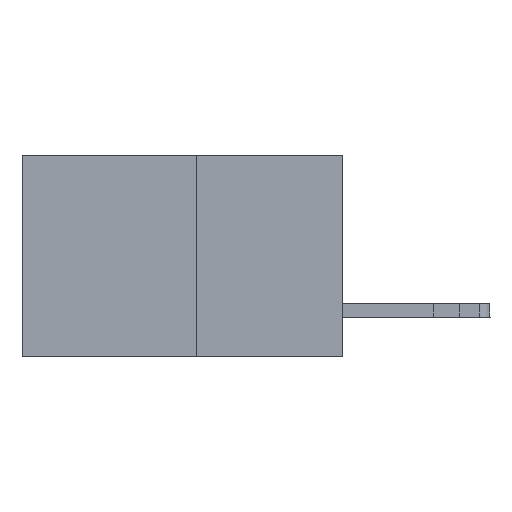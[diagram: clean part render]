
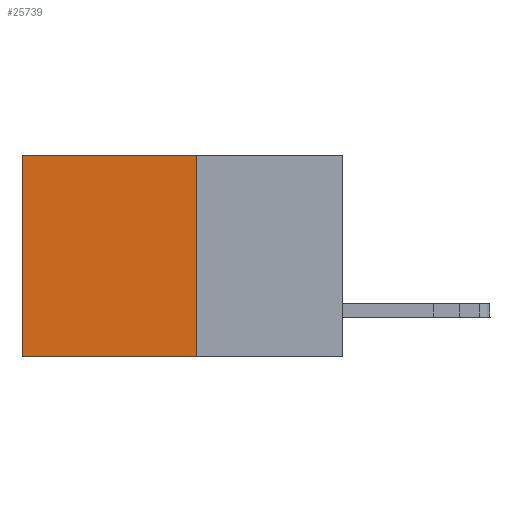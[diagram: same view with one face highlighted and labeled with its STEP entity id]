
A CAD part, left-side view. The second image highlights one B-rep face of the part: STEP entity #25739.
In plain terms, the highlighted planar face has unit normal (-1, 0, 0).
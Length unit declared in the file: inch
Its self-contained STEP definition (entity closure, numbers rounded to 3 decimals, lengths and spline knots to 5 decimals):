
#247 = CARTESIAN_POINT ( 'NONE',  ( 0.277, 0.27, -0.37 ) ) ;
#600 = CARTESIAN_POINT ( 'NONE',  ( 0.277, 0.27, -0.37 ) ) ;
#1344 = LINE ( 'NONE', #10391, #22843 ) ;
#1369 = EDGE_CURVE ( 'NONE', #4654, #6719, #7215, .T. ) ;
#2319 = ORIENTED_EDGE ( 'NONE', *, *, #10884, .F. ) ;
#2559 = DIRECTION ( 'NONE',  ( 0., 0., -1. ) ) ;
#2592 = EDGE_CURVE ( 'NONE', #15973, #8882, #1344, .T. ) ;
#3069 = VECTOR ( 'NONE', #20587, 39.37008 ) ;
#4654 = VERTEX_POINT ( 'NONE', #10740 ) ;
#5733 = EDGE_CURVE ( 'NONE', #4654, #15973, #11268, .T. ) ;
#6719 = VERTEX_POINT ( 'NONE', #23622 ) ;
#6954 = DIRECTION ( 'NONE',  ( 0., 1., 0. ) ) ;
#7006 = ORIENTED_EDGE ( 'NONE', *, *, #5733, .T. ) ;
#7215 = LINE ( 'NONE', #247, #3069 ) ;
#8288 = VECTOR ( 'NONE', #6954, 39.37008 ) ;
#8788 = FACE_OUTER_BOUND ( 'NONE', #15843, .T. ) ;
#8882 = VERTEX_POINT ( 'NONE', #25001 ) ;
#9645 = DIRECTION ( 'NONE',  ( 0., 1., 0. ) ) ;
#10391 = CARTESIAN_POINT ( 'NONE',  ( 0.277, 0.59, -0.37 ) ) ;
#10740 = CARTESIAN_POINT ( 'NONE',  ( 0.277, 0.27, 0. ) ) ;
#10884 = EDGE_CURVE ( 'NONE', #6719, #8882, #20947, .T. ) ;
#11110 = CARTESIAN_POINT ( 'NONE',  ( 0.277, 0.27, 0. ) ) ;
#11268 = LINE ( 'NONE', #11110, #8288 ) ;
#12710 = VECTOR ( 'NONE', #9645, 39.37008 ) ;
#15811 = ORIENTED_EDGE ( 'NONE', *, *, #2592, .T. ) ;
#15843 = EDGE_LOOP ( 'NONE', ( #15811, #2319, #28650, #7006 ) ) ;
#15973 = VERTEX_POINT ( 'NONE', #17455 ) ;
#17455 = CARTESIAN_POINT ( 'NONE',  ( 0.277, 0.59, 0. ) ) ;
#18154 = DIRECTION ( 'NONE',  ( 1., 0., 0. ) ) ;
#20587 = DIRECTION ( 'NONE',  ( 0., 0., -1. ) ) ;
#20947 = LINE ( 'NONE', #600, #12710 ) ;
#22673 = AXIS2_PLACEMENT_3D ( 'NONE', #25143, #18154, #2559 ) ;
#22758 = PLANE ( 'NONE',  #22673 ) ;
#22843 = VECTOR ( 'NONE', #28513, 39.37008 ) ;
#23622 = CARTESIAN_POINT ( 'NONE',  ( 0.277, 0.27, -0.37 ) ) ;
#25001 = CARTESIAN_POINT ( 'NONE',  ( 0.277, 0.59, -0.37 ) ) ;
#25143 = CARTESIAN_POINT ( 'NONE',  ( 0.277, 0.27, -0.37 ) ) ;
#25739 = ADVANCED_FACE ( 'NONE', ( #8788 ), #22758, .F. ) ;
#28513 = DIRECTION ( 'NONE',  ( 0., 0., -1. ) ) ;
#28650 = ORIENTED_EDGE ( 'NONE', *, *, #1369, .F. ) ;
